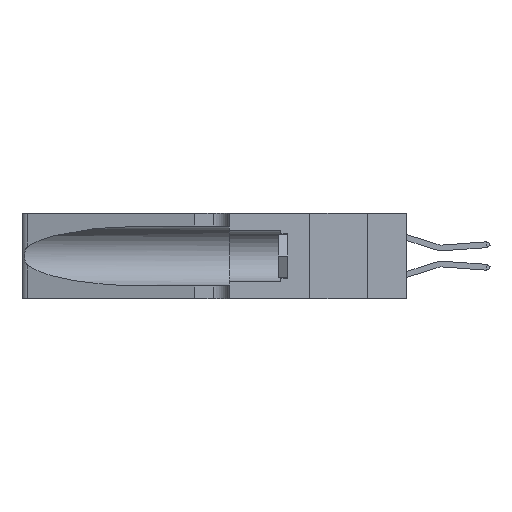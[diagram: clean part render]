
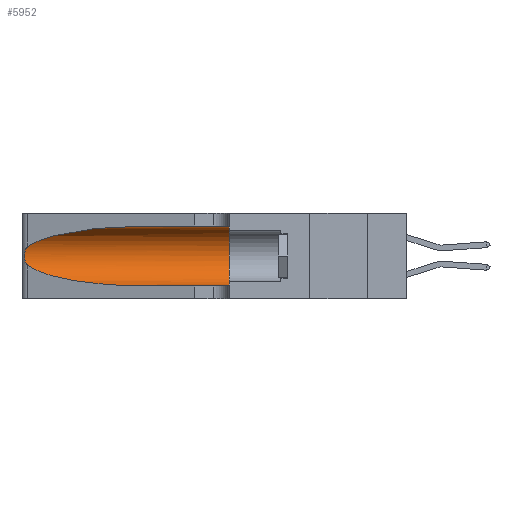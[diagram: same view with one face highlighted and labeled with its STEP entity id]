
A CAD part, left-side view. The second image highlights one B-rep face of the part: STEP entity #5952.
In plain terms, the highlighted cylindrical face has radius 3.308 mm (diameter 6.617 mm), a partial arc.
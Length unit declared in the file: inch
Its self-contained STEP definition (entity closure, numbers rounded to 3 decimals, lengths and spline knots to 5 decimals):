
#487 = CYLINDRICAL_SURFACE ( 'NONE', #10830, 0.13025 ) ;
#1227 = CARTESIAN_POINT ( 'NONE',  ( 0.25487, 1.22718, 0.14631 ) ) ;
#1966 = VERTEX_POINT ( 'NONE', #15684 ) ;
#2836 = AXIS2_PLACEMENT_3D ( 'NONE', #18755, #7242, #20645 ) ;
#3110 = CARTESIAN_POINT ( 'NONE',  ( 0.18966, 0.96281, 0.31525 ) ) ;
#3236 = CARTESIAN_POINT ( 'NONE',  ( 0.18966, 0.96281, 0.05475 ) ) ;
#3308 = CARTESIAN_POINT ( 'NONE',  ( 0.25787, 1.23484, 0.2124 ) ) ;
#5162 = CARTESIAN_POINT ( 'NONE',  ( 0.25487, 1.22718, 0.22369 ) ) ;
#5235 = CARTESIAN_POINT ( 'NONE',  ( 0.1305, 0.35, 0.31525 ) ) ;
#5293 = CARTESIAN_POINT ( 'NONE',  ( 0.26018, 1.23835, 0.19895 ) ) ;
#5926 = VERTEX_POINT ( 'NONE', #13193 ) ;
#5952 = ADVANCED_FACE ( 'NONE', ( #10973 ), #487, .F. ) ;
#6102 = CARTESIAN_POINT ( 'NONE',  ( 0.1305, 1.61858, 0.05475 ) ) ;
#6899 = ORIENTED_EDGE ( 'NONE', *, *, #24351, .T. ) ;
#6925 = EDGE_CURVE ( 'NONE', #5926, #21760, #17156, .T. ) ;
#7152 = ORIENTED_EDGE ( 'NONE', *, *, #19449, .F. ) ;
#7242 = DIRECTION ( 'NONE',  ( 0., 1., 0. ) ) ;
#7255 = CARTESIAN_POINT ( 'NONE',  ( 0.26075, 1.23896, 0.178 ) ) ;
#7437 = DIRECTION ( 'NONE',  ( 0., -1., 0. ) ) ;
#8322 = CARTESIAN_POINT ( 'NONE',  ( 0.1305, 1.61858, 0.31525 ) ) ;
#8836 = EDGE_CURVE ( 'NONE', #21760, #14170, #19343, .T. ) ;
#8923 = CARTESIAN_POINT ( 'NONE',  ( 0.25487, 1.22718, 0.14631 ) ) ;
#9051 = LINE ( 'NONE', #6102, #18584 ) ;
#9055 = ORIENTED_EDGE ( 'NONE', *, *, #21037, .F. ) ;
#9194 = CARTESIAN_POINT ( 'NONE',  ( 0.25487, 1.22718, 0.22369 ) ) ;
#9277 = CARTESIAN_POINT ( 'NONE',  ( 0.25856, 1.23593, 0.16098 ) ) ;
#9344 = ORIENTED_EDGE ( 'NONE', *, *, #9599, .T. ) ;
#9599 = EDGE_CURVE ( 'NONE', #14170, #17505, #9051, .T. ) ;
#10825 = CARTESIAN_POINT ( 'NONE',  ( 0.1305, 0.72297, 0.05475 ) ) ;
#10830 = AXIS2_PLACEMENT_3D ( 'NONE', #24531, #7437, #15142 ) ;
#10973 = FACE_OUTER_BOUND ( 'NONE', #11455, .T. ) ;
#11193 = CARTESIAN_POINT ( 'NONE',  ( 0.25639, 1.23186, 0.15144 ) ) ;
#11455 = EDGE_LOOP ( 'NONE', ( #6899, #16029, #21808, #9344, #7152, #9055 ) ) ;
#12190 = LINE ( 'NONE', #8322, #21642 ) ;
#12214 = DIRECTION ( 'NONE',  ( 0., -1., 0. ) ) ;
#12919 = CARTESIAN_POINT ( 'NONE',  ( 0.1305, 0.72297, 0.31525 ) ) ;
#13099 = CARTESIAN_POINT ( 'NONE',  ( 0.25487, 1.22718, 0.14631 ) ) ;
#13193 = CARTESIAN_POINT ( 'NONE',  ( 0.25487, 1.22718, 0.22369 ) ) ;
#13853 = DIRECTION ( 'NONE',  ( 0., -1., 0. ) ) ;
#14170 = VERTEX_POINT ( 'NONE', #10825 ) ;
#14335 =( BOUNDED_CURVE ( )  B_SPLINE_CURVE ( 3, ( #12919, #3110, #16752, #5162 ),
 .UNSPECIFIED., .F., .T. ) 
 B_SPLINE_CURVE_WITH_KNOTS ( ( 4, 4 ),
 ( 1.5708, 2.84003 ),
 .UNSPECIFIED. ) 
 CURVE ( )  GEOMETRIC_REPRESENTATION_ITEM ( )  RATIONAL_B_SPLINE_CURVE ( ( 1., 0.87, 0.87, 1. ) ) 
 REPRESENTATION_ITEM ( '' )  );
#14869 = CARTESIAN_POINT ( 'NONE',  ( 0.2373, 1.15595, 0.08982 ) ) ;
#14958 = CARTESIAN_POINT ( 'NONE',  ( 0.25639, 1.23184, 0.21858 ) ) ;
#15142 = DIRECTION ( 'NONE',  ( 0., 0., -1. ) ) ;
#15684 = CARTESIAN_POINT ( 'NONE',  ( 0.1305, 0.72297, 0.31525 ) ) ;
#15808 = VERTEX_POINT ( 'NONE', #5235 ) ;
#16029 = ORIENTED_EDGE ( 'NONE', *, *, #6925, .T. ) ;
#16749 = CIRCLE ( 'NONE', #2836, 0.13025 ) ;
#16752 = CARTESIAN_POINT ( 'NONE',  ( 0.2373, 1.15595, 0.28018 ) ) ;
#16790 = CARTESIAN_POINT ( 'NONE',  ( 0.1305, 0.72297, 0.05475 ) ) ;
#16860 = CARTESIAN_POINT ( 'NONE',  ( 0.25854, 1.2359, 0.20912 ) ) ;
#17156 = B_SPLINE_CURVE_WITH_KNOTS ( 'NONE', 3,
 ( #9194, #24357, #14958, #3308, #16860, #5293, #18772, #7255, #20657, #9277, #22538, #11193, #24448, #13099 ),
 .UNSPECIFIED., .F., .F.,
 ( 4, 2, 2, 2, 2, 2, 4 ),
 ( 0., 0.00027, 0.00053, 0.00107, 0.0016, 0.00187, 0.00214 ),
 .UNSPECIFIED. ) ;
#17505 = VERTEX_POINT ( 'NONE', #23987 ) ;
#18584 = VECTOR ( 'NONE', #13853, 39.37008 ) ;
#18755 = CARTESIAN_POINT ( 'NONE',  ( 0.1305, 0.35, 0.185 ) ) ;
#18772 = CARTESIAN_POINT ( 'NONE',  ( 0.26075, 1.23896, 0.19203 ) ) ;
#19343 =( BOUNDED_CURVE ( )  B_SPLINE_CURVE ( 3, ( #1227, #14869, #3236, #16790 ),
 .UNSPECIFIED., .F., .F. ) 
 B_SPLINE_CURVE_WITH_KNOTS ( ( 4, 4 ),
 ( 3.44316, 4.71239 ),
 .UNSPECIFIED. ) 
 CURVE ( )  GEOMETRIC_REPRESENTATION_ITEM ( )  RATIONAL_B_SPLINE_CURVE ( ( 1., 0.87, 0.87, 1. ) ) 
 REPRESENTATION_ITEM ( '' )  );
#19449 = EDGE_CURVE ( 'NONE', #15808, #17505, #16749, .T. ) ;
#20645 = DIRECTION ( 'NONE',  ( 0., 0., 1. ) ) ;
#20657 = CARTESIAN_POINT ( 'NONE',  ( 0.26017, 1.23833, 0.17102 ) ) ;
#21037 = EDGE_CURVE ( 'NONE', #1966, #15808, #12190, .T. ) ;
#21642 = VECTOR ( 'NONE', #12214, 39.37008 ) ;
#21760 = VERTEX_POINT ( 'NONE', #8923 ) ;
#21808 = ORIENTED_EDGE ( 'NONE', *, *, #8836, .T. ) ;
#22538 = CARTESIAN_POINT ( 'NONE',  ( 0.25789, 1.23486, 0.15765 ) ) ;
#23987 = CARTESIAN_POINT ( 'NONE',  ( 0.1305, 0.35, 0.05475 ) ) ;
#24351 = EDGE_CURVE ( 'NONE', #1966, #5926, #14335, .T. ) ;
#24357 = CARTESIAN_POINT ( 'NONE',  ( 0.25555, 1.22994, 0.2215 ) ) ;
#24448 = CARTESIAN_POINT ( 'NONE',  ( 0.25555, 1.22993, 0.14849 ) ) ;
#24531 = CARTESIAN_POINT ( 'NONE',  ( 0.1305, 1.61858, 0.185 ) ) ;
